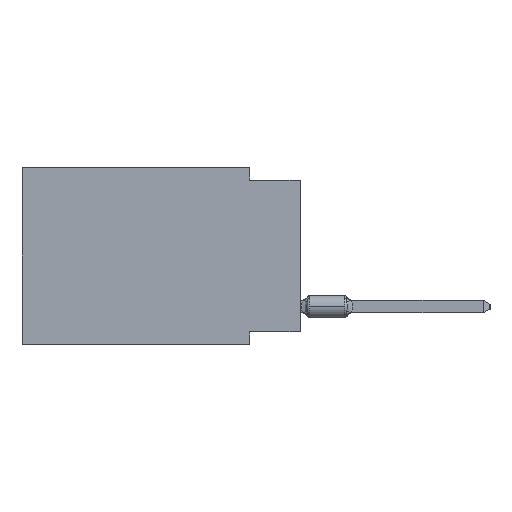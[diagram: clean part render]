
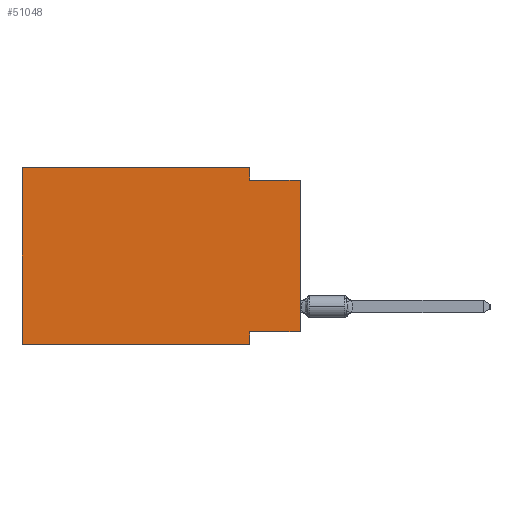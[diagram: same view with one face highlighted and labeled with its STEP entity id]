
A CAD part, left-side view. The second image highlights one B-rep face of the part: STEP entity #51048.
In plain terms, the highlighted planar face has unit normal (-1, 0, 0).
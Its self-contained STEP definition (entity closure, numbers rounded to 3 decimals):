
#1318 = VECTOR ( 'NONE', #25573, 1000. ) ;
#1766 = LINE ( 'NONE', #21025, #66748 ) ;
#4076 = ORIENTED_EDGE ( 'NONE', *, *, #49342, .F. ) ;
#5264 = ORIENTED_EDGE ( 'NONE', *, *, #30237, .F. ) ;
#6053 = CARTESIAN_POINT ( 'NONE',  ( 0., 2.54, -8.89 ) ) ;
#7890 = EDGE_CURVE ( 'NONE', #46517, #30492, #33410, .T. ) ;
#8893 = DIRECTION ( 'NONE',  ( 0., 0., -1. ) ) ;
#9428 = VERTEX_POINT ( 'NONE', #23688 ) ;
#10029 = EDGE_CURVE ( 'NONE', #46578, #30492, #64688, .T. ) ;
#11892 = VECTOR ( 'NONE', #38042, 1000. ) ;
#12950 = PLANE ( 'NONE',  #34763 ) ;
#13447 = LINE ( 'NONE', #34383, #47864 ) ;
#13586 = EDGE_CURVE ( 'NONE', #9428, #22271, #1766, .T. ) ;
#17682 = ORIENTED_EDGE ( 'NONE', *, *, #55128, .T. ) ;
#18404 = CARTESIAN_POINT ( 'NONE',  ( 0., 13.97, 0. ) ) ;
#19734 = DIRECTION ( 'NONE',  ( 0., 0., 1. ) ) ;
#20965 = VERTEX_POINT ( 'NONE', #69088 ) ;
#21025 = CARTESIAN_POINT ( 'NONE',  ( 0., 0., -0.635 ) ) ;
#22271 = VERTEX_POINT ( 'NONE', #45864 ) ;
#23688 = CARTESIAN_POINT ( 'NONE',  ( 0., 2.54, -0.635 ) ) ;
#25573 = DIRECTION ( 'NONE',  ( 0., 0., 1. ) ) ;
#26001 = CARTESIAN_POINT ( 'NONE',  ( 0., 2.54, -8.255 ) ) ;
#27341 = CARTESIAN_POINT ( 'NONE',  ( 0., 13.97, -8.89 ) ) ;
#29422 = LINE ( 'NONE', #59638, #68065 ) ;
#30237 = EDGE_CURVE ( 'NONE', #48222, #46517, #65655, .T. ) ;
#30492 = VERTEX_POINT ( 'NONE', #6053 ) ;
#33119 = CARTESIAN_POINT ( 'NONE',  ( 0., 13.97, -8.89 ) ) ;
#33410 = LINE ( 'NONE', #57752, #11892 ) ;
#34183 = CARTESIAN_POINT ( 'NONE',  ( 0., 0., -8.255 ) ) ;
#34383 = CARTESIAN_POINT ( 'NONE',  ( 0., 0., 0. ) ) ;
#34763 = AXIS2_PLACEMENT_3D ( 'NONE', #52362, #69591, #38519 ) ;
#38042 = DIRECTION ( 'NONE',  ( 0., 0., -1. ) ) ;
#38519 = DIRECTION ( 'NONE',  ( 0., 0., -1. ) ) ;
#40284 = EDGE_LOOP ( 'NONE', ( #17682, #53492, #56489, #79834, #4076, #52761, #44973, #5264 ) ) ;
#40483 = DIRECTION ( 'NONE',  ( 0., 1., 0. ) ) ;
#42711 = CARTESIAN_POINT ( 'NONE',  ( 0., 0., -8.255 ) ) ;
#44973 = ORIENTED_EDGE ( 'NONE', *, *, #7890, .F. ) ;
#45864 = CARTESIAN_POINT ( 'NONE',  ( 0., 0., -0.635 ) ) ;
#46517 = VERTEX_POINT ( 'NONE', #26001 ) ;
#46578 = VERTEX_POINT ( 'NONE', #33119 ) ;
#47563 = EDGE_CURVE ( 'NONE', #20965, #9428, #29422, .T. ) ;
#47864 = VECTOR ( 'NONE', #19734, 1000. ) ;
#48222 = VERTEX_POINT ( 'NONE', #42711 ) ;
#49342 = EDGE_CURVE ( 'NONE', #46578, #74042, #58689, .T. ) ;
#51048 = ADVANCED_FACE ( 'NONE', ( #64955 ), #12950, .F. ) ;
#51977 = CARTESIAN_POINT ( 'NONE',  ( 0., 13.97, 0. ) ) ;
#52362 = CARTESIAN_POINT ( 'NONE',  ( 0., 13.97, 0. ) ) ;
#52761 = ORIENTED_EDGE ( 'NONE', *, *, #10029, .T. ) ;
#53492 = ORIENTED_EDGE ( 'NONE', *, *, #13586, .F. ) ;
#55128 = EDGE_CURVE ( 'NONE', #48222, #22271, #13447, .T. ) ;
#56489 = ORIENTED_EDGE ( 'NONE', *, *, #47563, .F. ) ;
#57752 = CARTESIAN_POINT ( 'NONE',  ( 0., 2.54, -8.89 ) ) ;
#58689 = LINE ( 'NONE', #51977, #1318 ) ;
#59638 = CARTESIAN_POINT ( 'NONE',  ( 0., 2.54, 0. ) ) ;
#60223 = EDGE_CURVE ( 'NONE', #74042, #20965, #62039, .T. ) ;
#62039 = LINE ( 'NONE', #18404, #81745 ) ;
#64688 = LINE ( 'NONE', #27341, #80474 ) ;
#64955 = FACE_OUTER_BOUND ( 'NONE', #40284, .T. ) ;
#65099 = DIRECTION ( 'NONE',  ( 0., -1., 0. ) ) ;
#65655 = LINE ( 'NONE', #34183, #81662 ) ;
#65913 = DIRECTION ( 'NONE',  ( 0., -1., 0. ) ) ;
#66748 = VECTOR ( 'NONE', #65913, 1000. ) ;
#68065 = VECTOR ( 'NONE', #8893, 1000. ) ;
#69088 = CARTESIAN_POINT ( 'NONE',  ( 0., 2.54, 0. ) ) ;
#69591 = DIRECTION ( 'NONE',  ( 1., 0., 0. ) ) ;
#74042 = VERTEX_POINT ( 'NONE', #81661 ) ;
#79834 = ORIENTED_EDGE ( 'NONE', *, *, #60223, .F. ) ;
#80474 = VECTOR ( 'NONE', #65099, 1000. ) ;
#81330 = DIRECTION ( 'NONE',  ( 0., -1., 0. ) ) ;
#81662 = VECTOR ( 'NONE', #40483, 1000. ) ;
#81661 = CARTESIAN_POINT ( 'NONE',  ( 0., 13.97, 0. ) ) ;
#81745 = VECTOR ( 'NONE', #81330, 1000. ) ;
